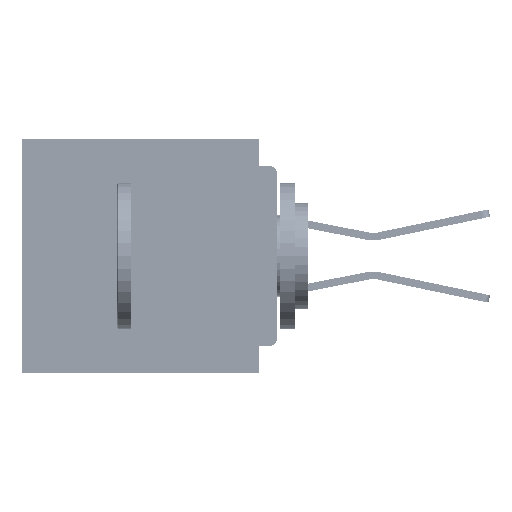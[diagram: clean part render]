
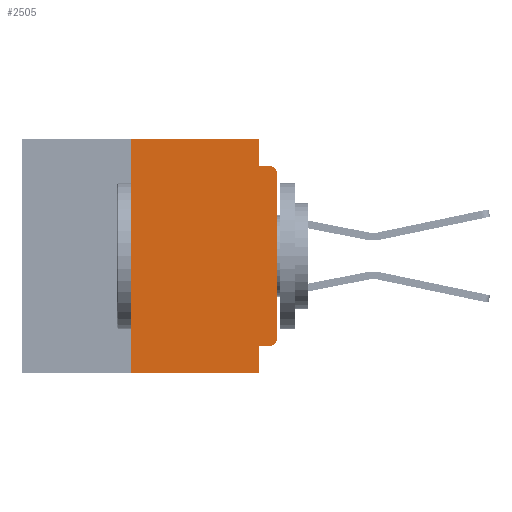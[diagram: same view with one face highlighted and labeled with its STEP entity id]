
A CAD part, left-side view. The second image highlights one B-rep face of the part: STEP entity #2505.
In plain terms, the highlighted planar face has unit normal (-1, 0, 0).
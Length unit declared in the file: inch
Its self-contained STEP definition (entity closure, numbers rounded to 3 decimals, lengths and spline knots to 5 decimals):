
#49 = VERTEX_POINT ( 'NONE', #27197 ) ;
#88 = CARTESIAN_POINT ( 'NONE',  ( 0., 0.437, -0.4 ) ) ;
#373 = LINE ( 'NONE', #9611, #29317 ) ;
#437 = CARTESIAN_POINT ( 'NONE',  ( 0., 0.015, -0.045 ) ) ;
#1068 = CARTESIAN_POINT ( 'NONE',  ( 0., 0.031, -0.355 ) ) ;
#1869 = CARTESIAN_POINT ( 'NONE',  ( 0., 0.437, 0. ) ) ;
#2505 = ADVANCED_FACE ( 'NONE', ( #67436 ), #40114, .F. ) ;
#3413 = ORIENTED_EDGE ( 'NONE', *, *, #41308, .F. ) ;
#4358 = EDGE_CURVE ( 'NONE', #64264, #6181, #45806, .T. ) ;
#4458 = AXIS2_PLACEMENT_3D ( 'NONE', #42892, #10404, #48366 ) ;
#4472 = LINE ( 'NONE', #20743, #29996 ) ;
#4548 = DIRECTION ( 'NONE',  ( 0., -1., 0. ) ) ;
#5088 = DIRECTION ( 'NONE',  ( 0., 0., 1. ) ) ;
#5822 = AXIS2_PLACEMENT_3D ( 'NONE', #17474, #55429, #22948 ) ;
#6181 = VERTEX_POINT ( 'NONE', #53725 ) ;
#7600 = DIRECTION ( 'NONE',  ( 1., 0., 0. ) ) ;
#7898 = LINE ( 'NONE', #13250, #49556 ) ;
#8783 = VECTOR ( 'NONE', #26904, 39.37008 ) ;
#8788 = EDGE_CURVE ( 'NONE', #32254, #30589, #4472, .T. ) ;
#9469 = VECTOR ( 'NONE', #54284, 39.37008 ) ;
#9611 = CARTESIAN_POINT ( 'NONE',  ( 0., 0.031, -0.4 ) ) ;
#10404 = DIRECTION ( 'NONE',  ( -1., 0., 0. ) ) ;
#11387 = ORIENTED_EDGE ( 'NONE', *, *, #57598, .T. ) ;
#12206 = DIRECTION ( 'NONE',  ( 0., 0., -1. ) ) ;
#13250 = CARTESIAN_POINT ( 'NONE',  ( 0., 0., -0.355 ) ) ;
#13259 = ORIENTED_EDGE ( 'NONE', *, *, #63849, .F. ) ;
#13538 = CARTESIAN_POINT ( 'NONE',  ( 0., 0.031, 0. ) ) ;
#15109 = DIRECTION ( 'NONE',  ( 0., 0., -1. ) ) ;
#15781 = ORIENTED_EDGE ( 'NONE', *, *, #68097, .F. ) ;
#16268 = LINE ( 'NONE', #70049, #43396 ) ;
#16545 = CARTESIAN_POINT ( 'NONE',  ( 0., 0., -0.34 ) ) ;
#16661 = VERTEX_POINT ( 'NONE', #53058 ) ;
#16948 = VECTOR ( 'NONE', #12206, 39.37008 ) ;
#17474 = CARTESIAN_POINT ( 'NONE',  ( 0., 0.015, -0.34 ) ) ;
#17892 = ORIENTED_EDGE ( 'NONE', *, *, #8788, .F. ) ;
#20053 = CIRCLE ( 'NONE', #4458, 0.015 ) ;
#20743 = CARTESIAN_POINT ( 'NONE',  ( 0., 0., -0.045 ) ) ;
#21709 = CIRCLE ( 'NONE', #5822, 0.015 ) ;
#22948 = DIRECTION ( 'NONE',  ( 0., 0., -1. ) ) ;
#23812 = EDGE_CURVE ( 'NONE', #36390, #32254, #31404, .T. ) ;
#25639 = LINE ( 'NONE', #88, #9469 ) ;
#26904 = DIRECTION ( 'NONE',  ( 0., -1., 0. ) ) ;
#27197 = CARTESIAN_POINT ( 'NONE',  ( 0., 0.25, 0. ) ) ;
#27555 = VERTEX_POINT ( 'NONE', #1068 ) ;
#29317 = VECTOR ( 'NONE', #15109, 39.37008 ) ;
#29996 = VECTOR ( 'NONE', #4548, 39.37008 ) ;
#30589 = VERTEX_POINT ( 'NONE', #437 ) ;
#30604 = ORIENTED_EDGE ( 'NONE', *, *, #67579, .T. ) ;
#31404 = LINE ( 'NONE', #33821, #16948 ) ;
#32254 = VERTEX_POINT ( 'NONE', #46479 ) ;
#32601 = ORIENTED_EDGE ( 'NONE', *, *, #23812, .F. ) ;
#33717 = ORIENTED_EDGE ( 'NONE', *, *, #68857, .F. ) ;
#33821 = CARTESIAN_POINT ( 'NONE',  ( 0., 0.031, 0. ) ) ;
#36390 = VERTEX_POINT ( 'NONE', #13538 ) ;
#37659 = LINE ( 'NONE', #37992, #8783 ) ;
#37992 = CARTESIAN_POINT ( 'NONE',  ( 0., 0.437, 0. ) ) ;
#40114 = PLANE ( 'NONE',  #63928 ) ;
#41308 = EDGE_CURVE ( 'NONE', #16661, #49, #16268, .T. ) ;
#42390 = VERTEX_POINT ( 'NONE', #42916 ) ;
#42892 = CARTESIAN_POINT ( 'NONE',  ( 0., 0.015, -0.06 ) ) ;
#42916 = CARTESIAN_POINT ( 'NONE',  ( 0., 0.015, -0.355 ) ) ;
#43396 = VECTOR ( 'NONE', #5088, 39.37008 ) ;
#44183 = EDGE_LOOP ( 'NONE', ( #46292, #30604, #17892, #32601, #33717, #3413, #60765, #15781, #13259, #11387 ) ) ;
#44874 = DIRECTION ( 'NONE',  ( 0., 0., 1. ) ) ;
#45607 = DIRECTION ( 'NONE',  ( 0., 0., -1. ) ) ;
#45806 = LINE ( 'NONE', #55785, #60268 ) ;
#46292 = ORIENTED_EDGE ( 'NONE', *, *, #4358, .T. ) ;
#46479 = CARTESIAN_POINT ( 'NONE',  ( 0., 0.031, -0.045 ) ) ;
#48366 = DIRECTION ( 'NONE',  ( 0., 0., -1. ) ) ;
#49556 = VECTOR ( 'NONE', #56653, 39.37008 ) ;
#53058 = CARTESIAN_POINT ( 'NONE',  ( 0., 0.25, -0.4 ) ) ;
#53413 = EDGE_CURVE ( 'NONE', #16661, #64238, #25639, .T. ) ;
#53725 = CARTESIAN_POINT ( 'NONE',  ( 0., 0., -0.06 ) ) ;
#54252 = CARTESIAN_POINT ( 'NONE',  ( 0., 0.031, -0.4 ) ) ;
#54284 = DIRECTION ( 'NONE',  ( 0., -1., 0. ) ) ;
#55429 = DIRECTION ( 'NONE',  ( -1., 0., 0. ) ) ;
#55785 = CARTESIAN_POINT ( 'NONE',  ( 0., 0., 0. ) ) ;
#56653 = DIRECTION ( 'NONE',  ( 0., 1., 0. ) ) ;
#57598 = EDGE_CURVE ( 'NONE', #42390, #64264, #21709, .T. ) ;
#60268 = VECTOR ( 'NONE', #44874, 39.37008 ) ;
#60765 = ORIENTED_EDGE ( 'NONE', *, *, #53413, .T. ) ;
#63849 = EDGE_CURVE ( 'NONE', #42390, #27555, #7898, .T. ) ;
#63928 = AXIS2_PLACEMENT_3D ( 'NONE', #1869, #7600, #45607 ) ;
#64238 = VERTEX_POINT ( 'NONE', #54252 ) ;
#64264 = VERTEX_POINT ( 'NONE', #16545 ) ;
#67436 = FACE_OUTER_BOUND ( 'NONE', #44183, .T. ) ;
#67579 = EDGE_CURVE ( 'NONE', #6181, #30589, #20053, .T. ) ;
#68097 = EDGE_CURVE ( 'NONE', #27555, #64238, #373, .T. ) ;
#68857 = EDGE_CURVE ( 'NONE', #49, #36390, #37659, .T. ) ;
#70049 = CARTESIAN_POINT ( 'NONE',  ( 0., 0.25, -0.4 ) ) ;
